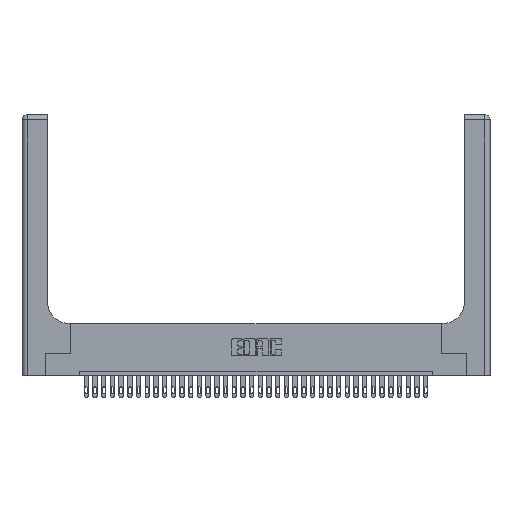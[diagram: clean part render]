
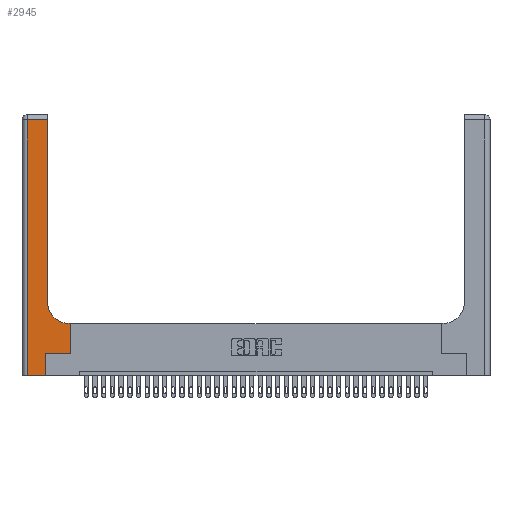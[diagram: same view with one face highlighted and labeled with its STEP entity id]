
A CAD part, top view. The second image highlights one B-rep face of the part: STEP entity #2945.
In plain terms, the highlighted planar face has unit normal (0, 0, 1).
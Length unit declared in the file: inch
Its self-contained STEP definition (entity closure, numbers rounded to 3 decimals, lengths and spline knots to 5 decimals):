
#599 = CARTESIAN_POINT ( 'NONE',  ( 0., 3., 0.37 ) ) ;
#649 = CARTESIAN_POINT ( 'NONE',  ( 0.5415, 0.85, 0.37 ) ) ;
#1225 = LINE ( 'NONE', #17338, #23026 ) ;
#2461 = EDGE_CURVE ( 'NONE', #6809, #12938, #4062, .T. ) ;
#2598 = LINE ( 'NONE', #9335, #23569 ) ;
#2641 = DIRECTION ( 'NONE',  ( 0., 1., 0. ) ) ;
#2945 = ADVANCED_FACE ( 'NONE', ( #30142 ), #30644, .F. ) ;
#3634 = CARTESIAN_POINT ( 'NONE',  ( 0.269, 0., 0.37 ) ) ;
#4062 = LINE ( 'NONE', #7588, #25421 ) ;
#5392 = EDGE_CURVE ( 'NONE', #27643, #30526, #2598, .T. ) ;
#6030 = LINE ( 'NONE', #21844, #26184 ) ;
#6463 = DIRECTION ( 'NONE',  ( 0., 1., 0. ) ) ;
#6753 = ORIENTED_EDGE ( 'NONE', *, *, #18619, .T. ) ;
#6809 = VERTEX_POINT ( 'NONE', #31243 ) ;
#7588 = CARTESIAN_POINT ( 'NONE',  ( 0.5585, 0.25, 0.37 ) ) ;
#7701 = LINE ( 'NONE', #19883, #33758 ) ;
#9073 = VERTEX_POINT ( 'NONE', #31135 ) ;
#9335 = CARTESIAN_POINT ( 'NONE',  ( 0., 0., 0.37 ) ) ;
#9619 = EDGE_CURVE ( 'NONE', #34880, #6809, #33954, .T. ) ;
#10176 = ORIENTED_EDGE ( 'NONE', *, *, #15399, .T. ) ;
#10515 = EDGE_CURVE ( 'NONE', #24385, #14415, #11658, .T. ) ;
#11249 = ORIENTED_EDGE ( 'NONE', *, *, #5392, .T. ) ;
#11658 = CIRCLE ( 'NONE', #20478, 0.25 ) ;
#12074 = ORIENTED_EDGE ( 'NONE', *, *, #10515, .T. ) ;
#12315 = ORIENTED_EDGE ( 'NONE', *, *, #16662, .T. ) ;
#12938 = VERTEX_POINT ( 'NONE', #15840 ) ;
#13195 = CARTESIAN_POINT ( 'NONE',  ( 0., 2.94, 0.37 ) ) ;
#14224 = DIRECTION ( 'NONE',  ( -1., 0., 0. ) ) ;
#14415 = VERTEX_POINT ( 'NONE', #14783 ) ;
#14522 = DIRECTION ( 'NONE',  ( 0., 0., -1. ) ) ;
#14783 = CARTESIAN_POINT ( 'NONE',  ( 0.2915, 0.85, 0.37 ) ) ;
#15085 = VECTOR ( 'NONE', #28754, 39.37008 ) ;
#15399 = EDGE_CURVE ( 'NONE', #30526, #34880, #28020, .T. ) ;
#15840 = CARTESIAN_POINT ( 'NONE',  ( 0.5585, 0.6, 0.37 ) ) ;
#16114 = DIRECTION ( 'NONE',  ( -1., 0., 0. ) ) ;
#16662 = EDGE_CURVE ( 'NONE', #9073, #23761, #23672, .T. ) ;
#17338 = CARTESIAN_POINT ( 'NONE',  ( 0.06, 3., 0.37 ) ) ;
#18619 = EDGE_CURVE ( 'NONE', #23761, #27643, #1225, .T. ) ;
#19310 = CARTESIAN_POINT ( 'NONE',  ( 0.269, 0., 0.37 ) ) ;
#19883 = CARTESIAN_POINT ( 'NONE',  ( 0.2915, 3., 0.37 ) ) ;
#19915 = DIRECTION ( 'NONE',  ( -1., 0., 0. ) ) ;
#20478 = AXIS2_PLACEMENT_3D ( 'NONE', #649, #14522, #25547 ) ;
#21844 = CARTESIAN_POINT ( 'NONE',  ( 0.2915, 0.6, 0.37 ) ) ;
#22338 = DIRECTION ( 'NONE',  ( 0., 0., -1. ) ) ;
#22786 = ORIENTED_EDGE ( 'NONE', *, *, #33349, .T. ) ;
#23026 = VECTOR ( 'NONE', #28303, 39.37008 ) ;
#23193 = CARTESIAN_POINT ( 'NONE',  ( 0.269, 0.25, 0.37 ) ) ;
#23569 = VECTOR ( 'NONE', #32066, 39.37008 ) ;
#23672 = LINE ( 'NONE', #13195, #25808 ) ;
#23761 = VERTEX_POINT ( 'NONE', #24868 ) ;
#24385 = VERTEX_POINT ( 'NONE', #34387 ) ;
#24868 = CARTESIAN_POINT ( 'NONE',  ( 0.06, 2.94, 0.37 ) ) ;
#25019 = CARTESIAN_POINT ( 'NONE',  ( 0.06, 0., 0.37 ) ) ;
#25021 = VECTOR ( 'NONE', #28296, 39.37008 ) ;
#25421 = VECTOR ( 'NONE', #2641, 39.37008 ) ;
#25547 = DIRECTION ( 'NONE',  ( 1., 0., 0. ) ) ;
#25808 = VECTOR ( 'NONE', #19915, 39.37008 ) ;
#26184 = VECTOR ( 'NONE', #16114, 39.37008 ) ;
#27643 = VERTEX_POINT ( 'NONE', #25019 ) ;
#28020 = LINE ( 'NONE', #3634, #25021 ) ;
#28296 = DIRECTION ( 'NONE',  ( 0., 1., 0. ) ) ;
#28303 = DIRECTION ( 'NONE',  ( 0., -1., 0. ) ) ;
#28754 = DIRECTION ( 'NONE',  ( 1., 0., 0. ) ) ;
#29226 = ORIENTED_EDGE ( 'NONE', *, *, #2461, .T. ) ;
#29298 = EDGE_LOOP ( 'NONE', ( #29902, #12315, #6753, #11249, #10176, #34701, #29226, #22786, #12074 ) ) ;
#29902 = ORIENTED_EDGE ( 'NONE', *, *, #32514, .T. ) ;
#29943 = AXIS2_PLACEMENT_3D ( 'NONE', #599, #22338, #14224 ) ;
#30142 = FACE_OUTER_BOUND ( 'NONE', #29298, .T. ) ;
#30526 = VERTEX_POINT ( 'NONE', #19310 ) ;
#30644 = PLANE ( 'NONE',  #29943 ) ;
#31135 = CARTESIAN_POINT ( 'NONE',  ( 0.2915, 2.94, 0.37 ) ) ;
#31243 = CARTESIAN_POINT ( 'NONE',  ( 0.5585, 0.25, 0.37 ) ) ;
#32066 = DIRECTION ( 'NONE',  ( 1., 0., 0. ) ) ;
#32514 = EDGE_CURVE ( 'NONE', #14415, #9073, #7701, .T. ) ;
#33349 = EDGE_CURVE ( 'NONE', #12938, #24385, #6030, .T. ) ;
#33758 = VECTOR ( 'NONE', #6463, 39.37008 ) ;
#33954 = LINE ( 'NONE', #34006, #15085 ) ;
#34006 = CARTESIAN_POINT ( 'NONE',  ( 0.269, 0.25, 0.37 ) ) ;
#34387 = CARTESIAN_POINT ( 'NONE',  ( 0.5415, 0.6, 0.37 ) ) ;
#34701 = ORIENTED_EDGE ( 'NONE', *, *, #9619, .T. ) ;
#34880 = VERTEX_POINT ( 'NONE', #23193 ) ;
